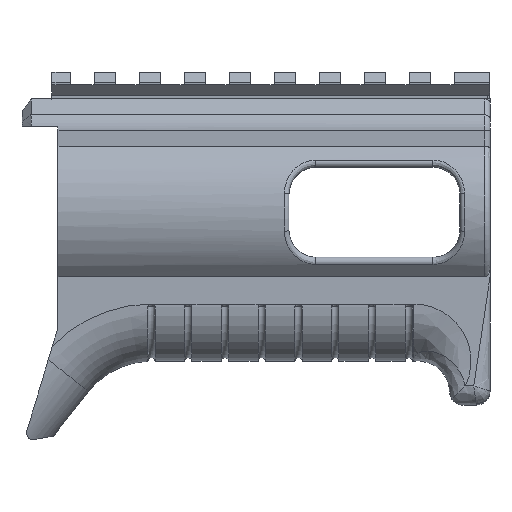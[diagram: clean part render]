
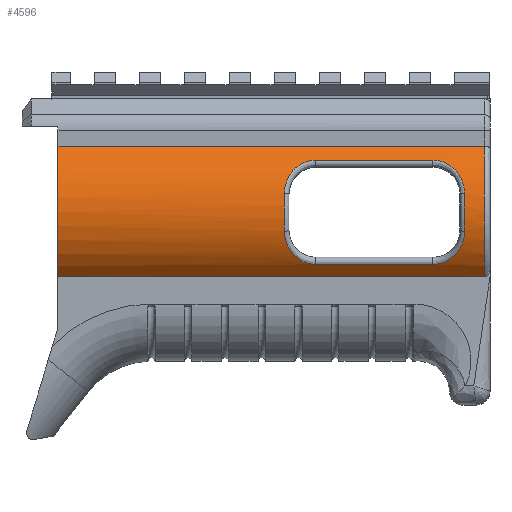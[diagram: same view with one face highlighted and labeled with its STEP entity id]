
A CAD part, left-side view. The second image highlights one B-rep face of the part: STEP entity #4596.
In plain terms, the highlighted cylindrical face has radius 20 mm (diameter 40 mm), a partial arc.
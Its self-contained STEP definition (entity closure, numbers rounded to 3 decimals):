
#114=CYLINDRICAL_SURFACE('',#4951,20.);
#159=B_SPLINE_CURVE_WITH_KNOTS('',3,(#7144,#7145,#7146,#7147,#7148,#7149,
#7150),.UNSPECIFIED.,.F.,.F.,(4,1,1,1,4),(0.,0.327,0.654,
0.981,1.145),.UNSPECIFIED.);
#161=B_SPLINE_CURVE_WITH_KNOTS('',3,(#7211,#7212,#7213,#7214,#7215,#7216,
#7217),.UNSPECIFIED.,.F.,.F.,(4,1,1,1,4),(0.,0.327,
0.491,0.818,1.145),.UNSPECIFIED.);
#163=B_SPLINE_CURVE_WITH_KNOTS('',3,(#7282,#7283,#7284,#7285,#7286,#7287,
#7288,#7289),.UNSPECIFIED.,.F.,.F.,(4,1,1,1,1,4),(0.,0.246,0.493,
0.821,0.985,1.149),.UNSPECIFIED.);
#165=B_SPLINE_CURVE_WITH_KNOTS('',3,(#7349,#7350,#7351,#7352,#7353,#7354,
#7355),.UNSPECIFIED.,.F.,.F.,(4,1,1,1,4),(0.,0.164,
0.493,0.821,1.149),.UNSPECIFIED.);
#288=FACE_BOUND('',#758,.T.);
#475=FACE_OUTER_BOUND('',#757,.T.);
#757=EDGE_LOOP('',(#3842,#3843,#3844,#3845));
#758=EDGE_LOOP('',(#3846,#3847,#3848,#3849,#3850,#3851,#3852,#3853));
#855=CIRCLE('',#4717,20.);
#880=CIRCLE('',#4853,20.);
#886=CIRCLE('',#4861,20.);
#927=CIRCLE('',#4952,20.);
#1264=LINE('',#7164,#1675);
#1266=LINE('',#7302,#1677);
#1340=LINE('',#8802,#1751);
#1341=LINE('',#8806,#1752);
#1675=VECTOR('',#5661,10.);
#1677=VECTOR('',#5679,10.);
#1751=VECTOR('',#5939,10.);
#1752=VECTOR('',#5944,10.);
#1825=VERTEX_POINT('',#6305);
#1826=VERTEX_POINT('',#6307);
#2020=VERTEX_POINT('',#7140);
#2022=VERTEX_POINT('',#7143);
#2024=VERTEX_POINT('',#7161);
#2026=VERTEX_POINT('',#7208);
#2028=VERTEX_POINT('',#7226);
#2030=VERTEX_POINT('',#7279);
#2032=VERTEX_POINT('',#7299);
#2034=VERTEX_POINT('',#7346);
#2124=VERTEX_POINT('',#8800);
#2125=VERTEX_POINT('',#8804);
#2239=EDGE_CURVE('',#1826,#1825,#855,.T.);
#2542=EDGE_CURVE('',#2022,#2020,#159,.T.);
#2546=EDGE_CURVE('',#2020,#2024,#1264,.T.);
#2549=EDGE_CURVE('',#2024,#2026,#161,.T.);
#2552=EDGE_CURVE('',#2026,#2028,#880,.T.);
#2555=EDGE_CURVE('',#2028,#2030,#163,.T.);
#2558=EDGE_CURVE('',#2030,#2032,#1266,.T.);
#2561=EDGE_CURVE('',#2032,#2034,#165,.T.);
#2564=EDGE_CURVE('',#2034,#2022,#886,.T.);
#2720=EDGE_CURVE('',#2124,#1826,#1340,.T.);
#2721=EDGE_CURVE('',#2124,#2125,#927,.T.);
#2722=EDGE_CURVE('',#1825,#2125,#1341,.T.);
#3842=ORIENTED_EDGE('',*,*,#2721,.F.);
#3843=ORIENTED_EDGE('',*,*,#2720,.T.);
#3844=ORIENTED_EDGE('',*,*,#2239,.T.);
#3845=ORIENTED_EDGE('',*,*,#2722,.T.);
#3846=ORIENTED_EDGE('',*,*,#2542,.T.);
#3847=ORIENTED_EDGE('',*,*,#2546,.T.);
#3848=ORIENTED_EDGE('',*,*,#2549,.T.);
#3849=ORIENTED_EDGE('',*,*,#2552,.T.);
#3850=ORIENTED_EDGE('',*,*,#2555,.T.);
#3851=ORIENTED_EDGE('',*,*,#2558,.T.);
#3852=ORIENTED_EDGE('',*,*,#2561,.T.);
#3853=ORIENTED_EDGE('',*,*,#2564,.T.);
#4596=ADVANCED_FACE('',(#475,#288),#114,.T.);
#4717=AXIS2_PLACEMENT_3D('',#6308,#5137,#5138);
#4853=AXIS2_PLACEMENT_3D('',#7229,#5669,#5670);
#4861=AXIS2_PLACEMENT_3D('',#7365,#5687,#5688);
#4951=AXIS2_PLACEMENT_3D('',#8803,#5940,#5941);
#4952=AXIS2_PLACEMENT_3D('',#8805,#5942,#5943);
#5137=DIRECTION('center_axis',(0.,-1.,0.));
#5138=DIRECTION('ref_axis',(0.,0.,
1.));
#5661=DIRECTION('',(0.,-1.,0.));
#5669=DIRECTION('center_axis',(0.,-1.,0.));
#5670=DIRECTION('ref_axis',(-1.,0.,-0.007));
#5679=DIRECTION('',(0.,1.,0.));
#5687=DIRECTION('center_axis',(0.,1.,0.));
#5688=DIRECTION('ref_axis',(-1.,0.,-0.007));
#5939=DIRECTION('',(0.,1.,0.));
#5940=DIRECTION('center_axis',(0.,-1.,0.));
#5941=DIRECTION('ref_axis',(0.,0.,
1.));
#5942=DIRECTION('center_axis',(0.,-1.,0.));
#5943=DIRECTION('ref_axis',(-1.,0.,0.));
#5944=DIRECTION('',(0.,-1.,0.));
#6305=CARTESIAN_POINT('',(-13.71,-131.348,-46.159));
#6307=CARTESIAN_POINT('',(-13.71,-131.348,-17.112));
#6308=CARTESIAN_POINT('Origin',(0.04,-131.348,-31.636));
#7140=CARTESIAN_POINT('',(-16.374,-188.68,-20.209));
#7143=CARTESIAN_POINT('',(-19.544,-181.68,-27.577));
#7144=CARTESIAN_POINT('Ctrl Pts',(-19.544,-181.68,-27.577));
#7145=CARTESIAN_POINT('Ctrl Pts',(-19.311,-181.68,-26.453));
#7146=CARTESIAN_POINT('Ctrl Pts',(-18.642,-182.179,-24.26));
#7147=CARTESIAN_POINT('Ctrl Pts',(-17.366,-184.104,-21.69));
#7148=CARTESIAN_POINT('Ctrl Pts',(-16.518,-186.495,-20.414));
#7149=CARTESIAN_POINT('Ctrl Pts',(-16.374,-188.135,-20.209));
#7150=CARTESIAN_POINT('Ctrl Pts',(-16.374,-188.68,-20.209));
#7161=CARTESIAN_POINT('',(-16.374,-214.68,-20.209));
#7164=CARTESIAN_POINT('',(-16.374,-227.348,-20.209));
#7208=CARTESIAN_POINT('',(-19.544,-221.68,-27.577));
#7211=CARTESIAN_POINT('Ctrl Pts',(-16.374,-214.68,-20.209));
#7212=CARTESIAN_POINT('Ctrl Pts',(-16.374,-215.771,-20.209));
#7213=CARTESIAN_POINT('Ctrl Pts',(-16.677,-217.388,-20.627));
#7214=CARTESIAN_POINT('Ctrl Pts',(-17.581,-219.572,-22.12));
#7215=CARTESIAN_POINT('Ctrl Pts',(-18.642,-221.183,-24.261));
#7216=CARTESIAN_POINT('Ctrl Pts',(-19.311,-221.68,-26.453));
#7217=CARTESIAN_POINT('Ctrl Pts',(-19.544,-221.68,-27.577));
#7226=CARTESIAN_POINT('',(-19.478,-221.68,-35.998));
#7229=CARTESIAN_POINT('Origin',(0.04,-221.68,-31.636));
#7279=CARTESIAN_POINT('',(-16.158,-214.68,-43.367));
#7282=CARTESIAN_POINT('Ctrl Pts',(-19.478,-221.68,-35.998));
#7283=CARTESIAN_POINT('Ctrl Pts',(-19.289,-221.68,-36.842));
#7284=CARTESIAN_POINT('Ctrl Pts',(-18.799,-221.402,-38.5));
#7285=CARTESIAN_POINT('Ctrl Pts',(-17.756,-220.15,-40.879));
#7286=CARTESIAN_POINT('Ctrl Pts',(-16.8,-218.338,-42.451));
#7287=CARTESIAN_POINT('Ctrl Pts',(-16.258,-216.321,-43.23));
#7288=CARTESIAN_POINT('Ctrl Pts',(-16.158,-215.228,-43.367));
#7289=CARTESIAN_POINT('Ctrl Pts',(-16.158,-214.68,-43.367));
#7299=CARTESIAN_POINT('',(-16.158,-188.68,-43.367));
#7302=CARTESIAN_POINT('',(-16.158,-227.348,-43.367));
#7346=CARTESIAN_POINT('',(-19.478,-181.68,-35.998));
#7349=CARTESIAN_POINT('Ctrl Pts',(-16.158,-188.68,-43.367));
#7350=CARTESIAN_POINT('Ctrl Pts',(-16.158,-188.133,-43.367));
#7351=CARTESIAN_POINT('Ctrl Pts',(-16.309,-186.487,-43.159));
#7352=CARTESIAN_POINT('Ctrl Pts',(-17.194,-184.098,-41.878));
#7353=CARTESIAN_POINT('Ctrl Pts',(-18.521,-182.179,-39.313));
#7354=CARTESIAN_POINT('Ctrl Pts',(-19.227,-181.68,-37.123));
#7355=CARTESIAN_POINT('Ctrl Pts',(-19.478,-181.68,-35.998));
#7365=CARTESIAN_POINT('Origin',(0.04,-181.68,-31.636));
#8800=CARTESIAN_POINT('',(-13.71,-226.078,-17.112));
#8802=CARTESIAN_POINT('',(-13.71,-227.348,-17.112));
#8803=CARTESIAN_POINT('Origin',(0.04,-227.348,-31.636));
#8804=CARTESIAN_POINT('',(-13.71,-226.078,-46.159));
#8805=CARTESIAN_POINT('Origin',(0.04,-226.078,-31.636));
#8806=CARTESIAN_POINT('',(-13.71,-227.348,-46.159));
